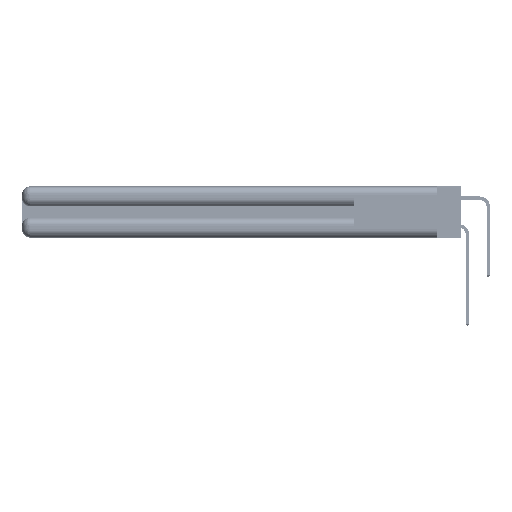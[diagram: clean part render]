
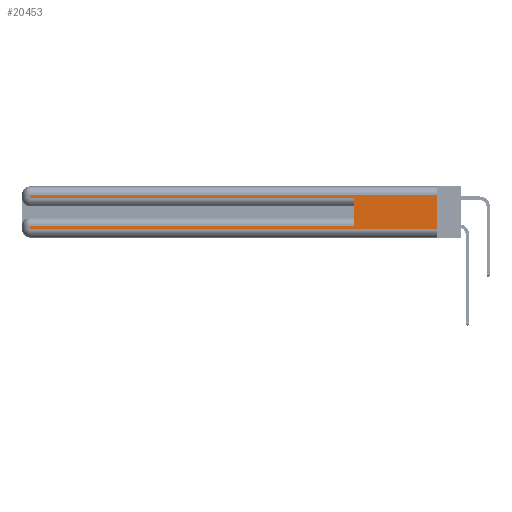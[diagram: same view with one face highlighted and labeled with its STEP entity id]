
A CAD part, left-side view. The second image highlights one B-rep face of the part: STEP entity #20453.
In plain terms, the highlighted planar face has unit normal (-1, 0, 0).
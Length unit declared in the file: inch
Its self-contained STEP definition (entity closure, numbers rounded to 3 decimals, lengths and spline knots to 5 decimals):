
#1015 = CARTESIAN_POINT ( 'NONE',  ( 0., 0., 0.085 ) ) ;
#1248 = DIRECTION ( 'NONE',  ( 1., 0., 0. ) ) ;
#1328 = EDGE_CURVE ( 'NONE', #11851, #41970, #45534, .T. ) ;
#1346 = CARTESIAN_POINT ( 'NONE',  ( 0., 2.94, 0.37 ) ) ;
#1438 = LINE ( 'NONE', #36126, #4641 ) ;
#2560 = CARTESIAN_POINT ( 'NONE',  ( 0., 2.94, 0.285 ) ) ;
#3777 = CARTESIAN_POINT ( 'NONE',  ( 0., 2.94, 0.31 ) ) ;
#3818 = EDGE_CURVE ( 'NONE', #28876, #8981, #45326, .T. ) ;
#4145 = VERTEX_POINT ( 'NONE', #29686 ) ;
#4641 = VECTOR ( 'NONE', #8013, 39.37008 ) ;
#4717 = CARTESIAN_POINT ( 'NONE',  ( 0., 0.6, 0.145 ) ) ;
#4826 = VERTEX_POINT ( 'NONE', #30600 ) ;
#7633 = ORIENTED_EDGE ( 'NONE', *, *, #1328, .T. ) ;
#8013 = DIRECTION ( 'NONE',  ( 0., 0., -1. ) ) ;
#8063 = ORIENTED_EDGE ( 'NONE', *, *, #15624, .T. ) ;
#8981 = VERTEX_POINT ( 'NONE', #48011 ) ;
#10778 = EDGE_CURVE ( 'NONE', #16996, #11851, #19270, .T. ) ;
#11548 = EDGE_CURVE ( 'NONE', #4145, #16996, #48579, .T. ) ;
#11851 = VERTEX_POINT ( 'NONE', #38462 ) ;
#12385 = LINE ( 'NONE', #4717, #16868 ) ;
#15624 = EDGE_CURVE ( 'NONE', #44181, #28876, #1438, .T. ) ;
#16868 = VECTOR ( 'NONE', #38004, 39.37008 ) ;
#16996 = VERTEX_POINT ( 'NONE', #21594 ) ;
#17391 = ORIENTED_EDGE ( 'NONE', *, *, #48923, .F. ) ;
#17892 = CARTESIAN_POINT ( 'NONE',  ( 0., 0., 0.37 ) ) ;
#18139 = CARTESIAN_POINT ( 'NONE',  ( 0., 0., 0.06 ) ) ;
#18340 = DIRECTION ( 'NONE',  ( 0., 0., -1. ) ) ;
#18351 = ORIENTED_EDGE ( 'NONE', *, *, #10778, .T. ) ;
#18421 = AXIS2_PLACEMENT_3D ( 'NONE', #17892, #1248, #50765 ) ;
#19270 = LINE ( 'NONE', #1346, #21160 ) ;
#20237 = CARTESIAN_POINT ( 'NONE',  ( 0., 0., 0.285 ) ) ;
#20453 = ADVANCED_FACE ( 'NONE', ( #48134 ), #50398, .F. ) ;
#21160 = VECTOR ( 'NONE', #18340, 39.37008 ) ;
#21594 = CARTESIAN_POINT ( 'NONE',  ( 0., 2.94, 0.085 ) ) ;
#22374 = ORIENTED_EDGE ( 'NONE', *, *, #3818, .T. ) ;
#23026 = DIRECTION ( 'NONE',  ( 0., 0., -1. ) ) ;
#26657 = EDGE_CURVE ( 'NONE', #4145, #8981, #12385, .T. ) ;
#28876 = VERTEX_POINT ( 'NONE', #2560 ) ;
#29686 = CARTESIAN_POINT ( 'NONE',  ( 0., 0.6, 0.085 ) ) ;
#30539 = DIRECTION ( 'NONE',  ( 0., 1., 0. ) ) ;
#30600 = CARTESIAN_POINT ( 'NONE',  ( 0., 0., 0.31 ) ) ;
#30826 = LINE ( 'NONE', #47468, #45482 ) ;
#31413 = ORIENTED_EDGE ( 'NONE', *, *, #40158, .T. ) ;
#32625 = VECTOR ( 'NONE', #40871, 39.37008 ) ;
#33570 = CARTESIAN_POINT ( 'NONE',  ( 0., 0., 0.31 ) ) ;
#36126 = CARTESIAN_POINT ( 'NONE',  ( 0., 2.94, 0.37 ) ) ;
#36463 = VECTOR ( 'NONE', #40780, 39.37008 ) ;
#38004 = DIRECTION ( 'NONE',  ( 0., 0., 1. ) ) ;
#38462 = CARTESIAN_POINT ( 'NONE',  ( 0., 2.94, 0.06 ) ) ;
#40158 = EDGE_CURVE ( 'NONE', #4826, #44181, #44617, .T. ) ;
#40780 = DIRECTION ( 'NONE',  ( 0., -1., 0. ) ) ;
#40871 = DIRECTION ( 'NONE',  ( 0., 1., 0. ) ) ;
#41970 = VERTEX_POINT ( 'NONE', #18139 ) ;
#44072 = DIRECTION ( 'NONE',  ( 0., -1., 0. ) ) ;
#44181 = VERTEX_POINT ( 'NONE', #3777 ) ;
#44617 = LINE ( 'NONE', #33570, #45899 ) ;
#45000 = ORIENTED_EDGE ( 'NONE', *, *, #26657, .F. ) ;
#45326 = LINE ( 'NONE', #20237, #36463 ) ;
#45482 = VECTOR ( 'NONE', #23026, 39.37008 ) ;
#45534 = LINE ( 'NONE', #51606, #52592 ) ;
#45899 = VECTOR ( 'NONE', #30539, 39.37008 ) ;
#47468 = CARTESIAN_POINT ( 'NONE',  ( 0., 0., 0.37 ) ) ;
#47697 = ORIENTED_EDGE ( 'NONE', *, *, #11548, .T. ) ;
#48011 = CARTESIAN_POINT ( 'NONE',  ( 0., 0.6, 0.285 ) ) ;
#48134 = FACE_OUTER_BOUND ( 'NONE', #51592, .T. ) ;
#48579 = LINE ( 'NONE', #1015, #32625 ) ;
#48923 = EDGE_CURVE ( 'NONE', #4826, #41970, #30826, .T. ) ;
#50398 = PLANE ( 'NONE',  #18421 ) ;
#50765 = DIRECTION ( 'NONE',  ( 0., 0., -1. ) ) ;
#51592 = EDGE_LOOP ( 'NONE', ( #17391, #31413, #8063, #22374, #45000, #47697, #18351, #7633 ) ) ;
#51606 = CARTESIAN_POINT ( 'NONE',  ( 0., 0., 0.06 ) ) ;
#52592 = VECTOR ( 'NONE', #44072, 39.37008 ) ;
